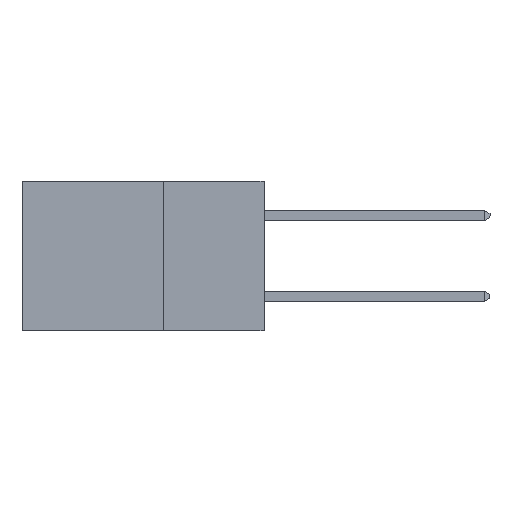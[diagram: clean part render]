
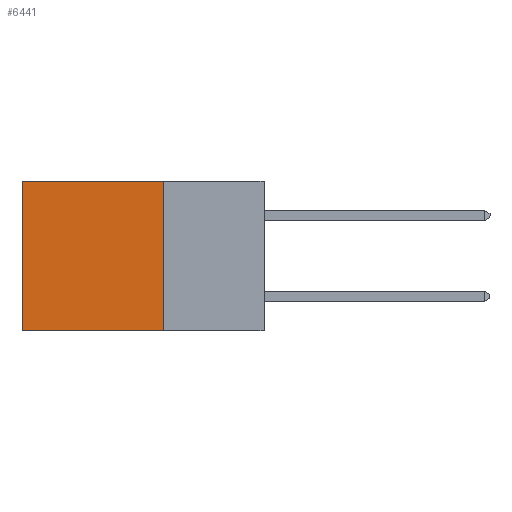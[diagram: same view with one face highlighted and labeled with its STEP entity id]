
A CAD part, left-side view. The second image highlights one B-rep face of the part: STEP entity #6441.
In plain terms, the highlighted planar face has unit normal (-1, 0, 0).
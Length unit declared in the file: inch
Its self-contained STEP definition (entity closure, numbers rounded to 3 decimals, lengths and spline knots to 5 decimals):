
#399 = EDGE_CURVE ( 'NONE', #5947, #6413, #8732, .T. ) ;
#672 = PLANE ( 'NONE',  #8796 ) ;
#936 = ORIENTED_EDGE ( 'NONE', *, *, #8520, .T. ) ;
#1014 = CARTESIAN_POINT ( 'NONE',  ( 0.298, 0.25, -0.37 ) ) ;
#1382 = VECTOR ( 'NONE', #1884, 39.37008 ) ;
#1491 = EDGE_LOOP ( 'NONE', ( #4710, #4966, #8790, #936 ) ) ;
#1659 = DIRECTION ( 'NONE',  ( 1., 0., 0. ) ) ;
#1884 = DIRECTION ( 'NONE',  ( 0., 0., -1. ) ) ;
#1985 = CARTESIAN_POINT ( 'NONE',  ( 0.298, 0.25, 0. ) ) ;
#3270 = EDGE_CURVE ( 'NONE', #6413, #9372, #6668, .T. ) ;
#3639 = LINE ( 'NONE', #11211, #1382 ) ;
#3912 = FACE_OUTER_BOUND ( 'NONE', #1491, .T. ) ;
#3984 = DIRECTION ( 'NONE',  ( 0., 1., 0. ) ) ;
#4183 = VERTEX_POINT ( 'NONE', #6836 ) ;
#4381 = VECTOR ( 'NONE', #3984, 39.37008 ) ;
#4547 = VECTOR ( 'NONE', #9584, 39.37008 ) ;
#4710 = ORIENTED_EDGE ( 'NONE', *, *, #8358, .T. ) ;
#4944 = CARTESIAN_POINT ( 'NONE',  ( 0.298, 0.25, -0.37 ) ) ;
#4966 = ORIENTED_EDGE ( 'NONE', *, *, #3270, .F. ) ;
#5699 = CARTESIAN_POINT ( 'NONE',  ( 0.298, 0.25, 0. ) ) ;
#5772 = CARTESIAN_POINT ( 'NONE',  ( 0.298, 0.6, -0.37 ) ) ;
#5947 = VERTEX_POINT ( 'NONE', #9543 ) ;
#6339 = DIRECTION ( 'NONE',  ( 0., 0., -1. ) ) ;
#6413 = VERTEX_POINT ( 'NONE', #4944 ) ;
#6441 = ADVANCED_FACE ( 'NONE', ( #3912 ), #672, .F. ) ;
#6668 = LINE ( 'NONE', #1014, #4381 ) ;
#6836 = CARTESIAN_POINT ( 'NONE',  ( 0.298, 0.6, 0. ) ) ;
#6839 = LINE ( 'NONE', #1985, #4547 ) ;
#7582 = DIRECTION ( 'NONE',  ( 0., 0., -1. ) ) ;
#8358 = EDGE_CURVE ( 'NONE', #4183, #9372, #3639, .T. ) ;
#8474 = VECTOR ( 'NONE', #6339, 39.37008 ) ;
#8520 = EDGE_CURVE ( 'NONE', #5947, #4183, #6839, .T. ) ;
#8732 = LINE ( 'NONE', #5699, #8474 ) ;
#8790 = ORIENTED_EDGE ( 'NONE', *, *, #399, .F. ) ;
#8796 = AXIS2_PLACEMENT_3D ( 'NONE', #10951, #1659, #7582 ) ;
#9372 = VERTEX_POINT ( 'NONE', #5772 ) ;
#9543 = CARTESIAN_POINT ( 'NONE',  ( 0.298, 0.25, 0. ) ) ;
#9584 = DIRECTION ( 'NONE',  ( 0., 1., 0. ) ) ;
#10951 = CARTESIAN_POINT ( 'NONE',  ( 0.298, 0.25, 0. ) ) ;
#11211 = CARTESIAN_POINT ( 'NONE',  ( 0.298, 0.6, 0. ) ) ;
